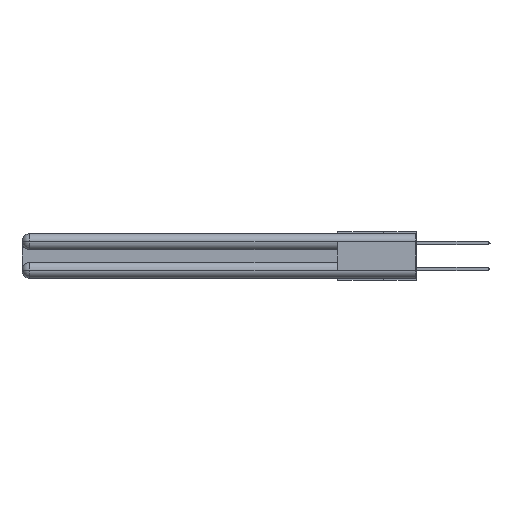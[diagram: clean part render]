
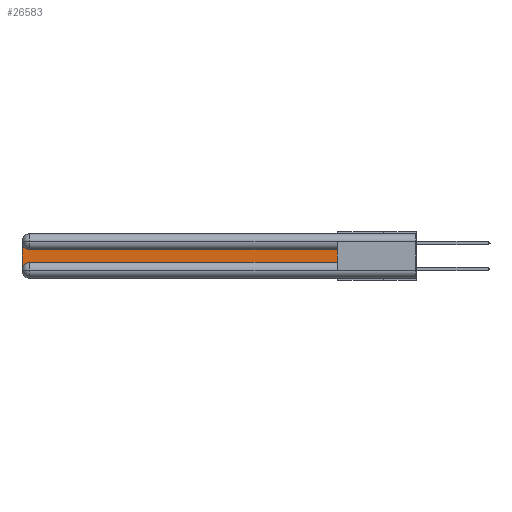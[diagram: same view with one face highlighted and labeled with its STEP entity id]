
A CAD part, left-side view. The second image highlights one B-rep face of the part: STEP entity #26583.
In plain terms, the highlighted planar face has unit normal (-1, 0, 0).
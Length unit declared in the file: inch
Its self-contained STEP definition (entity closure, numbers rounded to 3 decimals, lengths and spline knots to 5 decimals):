
#452 = CARTESIAN_POINT ( 'NONE',  ( 0.075, 0.6, -0.2175 ) ) ;
#756 = ORIENTED_EDGE ( 'NONE', *, *, #13254, .T. ) ;
#768 = CARTESIAN_POINT ( 'NONE',  ( 0.075, 3., -0.0625 ) ) ;
#1338 = CARTESIAN_POINT ( 'NONE',  ( 0.075, 2.94, -0.2175 ) ) ;
#1868 = CIRCLE ( 'NONE', #6042, 0.06 ) ;
#2136 = ORIENTED_EDGE ( 'NONE', *, *, #5401, .T. ) ;
#2788 = DIRECTION ( 'NONE',  ( 1., 0., 0. ) ) ;
#3373 = VECTOR ( 'NONE', #21208, 39.37008 ) ;
#3557 = CARTESIAN_POINT ( 'NONE',  ( 0.075, 3., -0.2175 ) ) ;
#5401 = EDGE_CURVE ( 'NONE', #26637, #21476, #28554, .T. ) ;
#5910 = AXIS2_PLACEMENT_3D ( 'NONE', #22032, #2788, #10192 ) ;
#6042 = AXIS2_PLACEMENT_3D ( 'NONE', #14055, #13646, #6332 ) ;
#6332 = DIRECTION ( 'NONE',  ( 0., 0., -1. ) ) ;
#8998 = CARTESIAN_POINT ( 'NONE',  ( 0.075, 3., -0.2775 ) ) ;
#9266 = FACE_OUTER_BOUND ( 'NONE', #24024, .T. ) ;
#9663 = VECTOR ( 'NONE', #21515, 39.37008 ) ;
#9806 = ORIENTED_EDGE ( 'NONE', *, *, #11613, .T. ) ;
#10192 = DIRECTION ( 'NONE',  ( 0., 0., -1. ) ) ;
#11613 = EDGE_CURVE ( 'NONE', #21736, #12961, #1868, .T. ) ;
#12486 = ORIENTED_EDGE ( 'NONE', *, *, #26610, .T. ) ;
#12801 = LINE ( 'NONE', #25611, #20722 ) ;
#12961 = VERTEX_POINT ( 'NONE', #768 ) ;
#13116 = CARTESIAN_POINT ( 'NONE',  ( 0.075, 0.6, -0.1225 ) ) ;
#13254 = EDGE_CURVE ( 'NONE', #21476, #25134, #12801, .T. ) ;
#13484 = CARTESIAN_POINT ( 'NONE',  ( 0.075, 2.94, -0.1225 ) ) ;
#13582 = DIRECTION ( 'NONE',  ( 0., 0., -1. ) ) ;
#13646 = DIRECTION ( 'NONE',  ( 1., 0., 0. ) ) ;
#14055 = CARTESIAN_POINT ( 'NONE',  ( 0.075, 2.94, -0.0625 ) ) ;
#15622 = AXIS2_PLACEMENT_3D ( 'NONE', #25605, #28030, #13582 ) ;
#19699 = PLANE ( 'NONE',  #5910 ) ;
#20167 = ORIENTED_EDGE ( 'NONE', *, *, #27492, .T. ) ;
#20482 = DIRECTION ( 'NONE',  ( 0., 1., 0. ) ) ;
#20522 = CIRCLE ( 'NONE', #15622, 0.06 ) ;
#20722 = VECTOR ( 'NONE', #28039, 39.37008 ) ;
#20821 = VERTEX_POINT ( 'NONE', #8998 ) ;
#21208 = DIRECTION ( 'NONE',  ( 0., 0., -1. ) ) ;
#21476 = VERTEX_POINT ( 'NONE', #452 ) ;
#21515 = DIRECTION ( 'NONE',  ( 0., -1., 0. ) ) ;
#21736 = VERTEX_POINT ( 'NONE', #13484 ) ;
#22032 = CARTESIAN_POINT ( 'NONE',  ( 0.075, 3., -0.1225 ) ) ;
#23534 = CARTESIAN_POINT ( 'NONE',  ( 0.075, 0.6, -0.2175 ) ) ;
#23998 = LINE ( 'NONE', #13116, #26249 ) ;
#24024 = EDGE_LOOP ( 'NONE', ( #12486, #9806, #26312, #20167, #2136, #756 ) ) ;
#25134 = VERTEX_POINT ( 'NONE', #28922 ) ;
#25605 = CARTESIAN_POINT ( 'NONE',  ( 0.075, 2.94, -0.2775 ) ) ;
#25611 = CARTESIAN_POINT ( 'NONE',  ( 0.075, 0.6, -0.2175 ) ) ;
#26249 = VECTOR ( 'NONE', #20482, 39.37008 ) ;
#26312 = ORIENTED_EDGE ( 'NONE', *, *, #30706, .T. ) ;
#26583 = ADVANCED_FACE ( 'NONE', ( #9266 ), #19699, .F. ) ;
#26610 = EDGE_CURVE ( 'NONE', #25134, #21736, #23998, .T. ) ;
#26637 = VERTEX_POINT ( 'NONE', #1338 ) ;
#26795 = LINE ( 'NONE', #3557, #3373 ) ;
#27492 = EDGE_CURVE ( 'NONE', #20821, #26637, #20522, .T. ) ;
#28030 = DIRECTION ( 'NONE',  ( 1., 0., 0. ) ) ;
#28039 = DIRECTION ( 'NONE',  ( 0., 0., 1. ) ) ;
#28554 = LINE ( 'NONE', #23534, #9663 ) ;
#28922 = CARTESIAN_POINT ( 'NONE',  ( 0.075, 0.6, -0.1225 ) ) ;
#30706 = EDGE_CURVE ( 'NONE', #12961, #20821, #26795, .T. ) ;
